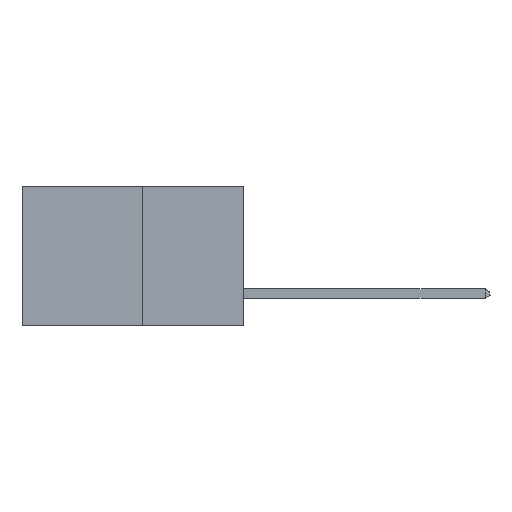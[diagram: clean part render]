
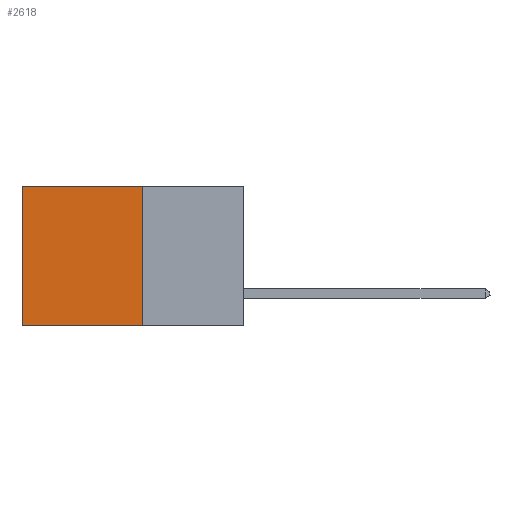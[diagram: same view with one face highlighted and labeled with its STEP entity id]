
A CAD part, left-side view. The second image highlights one B-rep face of the part: STEP entity #2618.
In plain terms, the highlighted planar face has unit normal (-1, 0, 0).
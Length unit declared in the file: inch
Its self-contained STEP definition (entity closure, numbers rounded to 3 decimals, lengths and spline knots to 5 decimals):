
#132 = CARTESIAN_POINT ( 'NONE',  ( 0.277, 0.27, 0. ) ) ;
#225 = DIRECTION ( 'NONE',  ( 0., 1., 0. ) ) ;
#238 = VECTOR ( 'NONE', #5093, 39.37008 ) ;
#1107 = ORIENTED_EDGE ( 'NONE', *, *, #6087, .F. ) ;
#2554 = CARTESIAN_POINT ( 'NONE',  ( 0.277, 0.27, 0. ) ) ;
#2587 = DIRECTION ( 'NONE',  ( 0., 1., 0. ) ) ;
#2618 = ADVANCED_FACE ( 'NONE', ( #7948 ), #8752, .F. ) ;
#2695 = LINE ( 'NONE', #4149, #4750 ) ;
#2984 = EDGE_CURVE ( 'NONE', #9145, #3614, #2695, .T. ) ;
#3451 = VERTEX_POINT ( 'NONE', #6192 ) ;
#3614 = VERTEX_POINT ( 'NONE', #6218 ) ;
#3898 = EDGE_LOOP ( 'NONE', ( #9114, #7218, #1107, #8736 ) ) ;
#4149 = CARTESIAN_POINT ( 'NONE',  ( 0.277, 0.27, -0.37 ) ) ;
#4584 = VECTOR ( 'NONE', #2587, 39.37008 ) ;
#4750 = VECTOR ( 'NONE', #225, 39.37008 ) ;
#4824 = LINE ( 'NONE', #7630, #6327 ) ;
#5070 = CARTESIAN_POINT ( 'NONE',  ( 0.277, 0.59, -0.37 ) ) ;
#5093 = DIRECTION ( 'NONE',  ( 0., 0., -1. ) ) ;
#6075 = EDGE_CURVE ( 'NONE', #8935, #3451, #6558, .T. ) ;
#6087 = EDGE_CURVE ( 'NONE', #8935, #9145, #4824, .T. ) ;
#6192 = CARTESIAN_POINT ( 'NONE',  ( 0.277, 0.59, 0. ) ) ;
#6218 = CARTESIAN_POINT ( 'NONE',  ( 0.277, 0.59, -0.37 ) ) ;
#6327 = VECTOR ( 'NONE', #6585, 39.37008 ) ;
#6423 = LINE ( 'NONE', #5070, #238 ) ;
#6558 = LINE ( 'NONE', #2554, #4584 ) ;
#6585 = DIRECTION ( 'NONE',  ( 0., 0., -1. ) ) ;
#6607 = AXIS2_PLACEMENT_3D ( 'NONE', #7653, #7100, #9050 ) ;
#7100 = DIRECTION ( 'NONE',  ( 1., 0., 0. ) ) ;
#7158 = EDGE_CURVE ( 'NONE', #3451, #3614, #6423, .T. ) ;
#7218 = ORIENTED_EDGE ( 'NONE', *, *, #2984, .F. ) ;
#7630 = CARTESIAN_POINT ( 'NONE',  ( 0.277, 0.27, -0.37 ) ) ;
#7653 = CARTESIAN_POINT ( 'NONE',  ( 0.277, 0.27, -0.37 ) ) ;
#7948 = FACE_OUTER_BOUND ( 'NONE', #3898, .T. ) ;
#7991 = CARTESIAN_POINT ( 'NONE',  ( 0.277, 0.27, -0.37 ) ) ;
#8736 = ORIENTED_EDGE ( 'NONE', *, *, #6075, .T. ) ;
#8752 = PLANE ( 'NONE',  #6607 ) ;
#8935 = VERTEX_POINT ( 'NONE', #132 ) ;
#9050 = DIRECTION ( 'NONE',  ( 0., 0., -1. ) ) ;
#9114 = ORIENTED_EDGE ( 'NONE', *, *, #7158, .T. ) ;
#9145 = VERTEX_POINT ( 'NONE', #7991 ) ;
